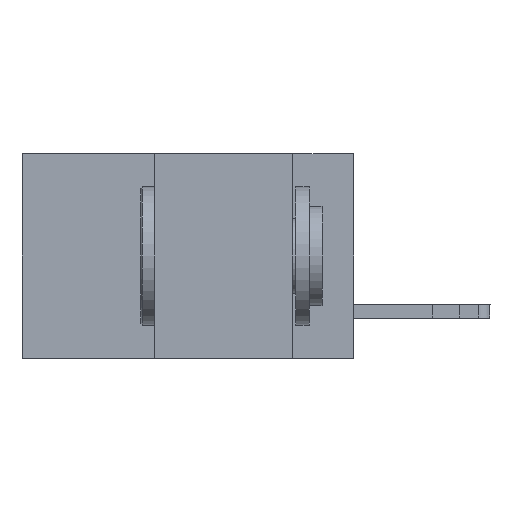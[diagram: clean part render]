
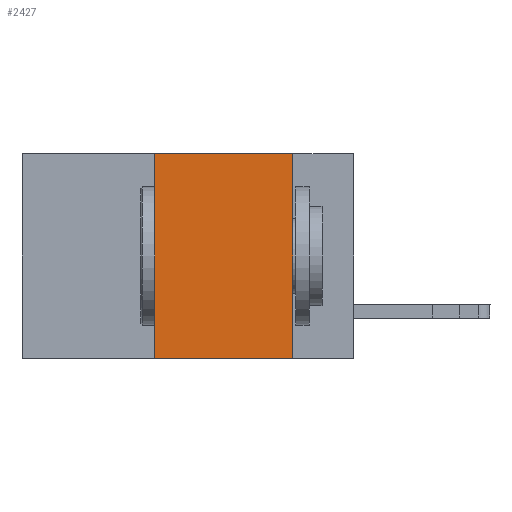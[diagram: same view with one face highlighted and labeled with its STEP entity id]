
A CAD part, left-side view. The second image highlights one B-rep face of the part: STEP entity #2427.
In plain terms, the highlighted planar face has unit normal (-1, 0, 0).
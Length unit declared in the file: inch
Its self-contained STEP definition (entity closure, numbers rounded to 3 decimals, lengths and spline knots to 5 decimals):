
#285 = DIRECTION ( 'NONE',  ( 0., 0., -1. ) ) ;
#447 = CARTESIAN_POINT ( 'NONE',  ( 0., 0.6, 0. ) ) ;
#644 = DIRECTION ( 'NONE',  ( 0., -1., 0. ) ) ;
#1502 = CARTESIAN_POINT ( 'NONE',  ( 0., 0.36, 0. ) ) ;
#1856 = EDGE_CURVE ( 'NONE', #11914, #11080, #3003, .T. ) ;
#2427 = ADVANCED_FACE ( 'NONE', ( #10348 ), #2671, .F. ) ;
#2671 = PLANE ( 'NONE',  #8887 ) ;
#3003 = LINE ( 'NONE', #12328, #4125 ) ;
#3534 = EDGE_LOOP ( 'NONE', ( #3798, #7673, #7021, #14537 ) ) ;
#3798 = ORIENTED_EDGE ( 'NONE', *, *, #1856, .F. ) ;
#3983 = EDGE_CURVE ( 'NONE', #14549, #11914, #4988, .T. ) ;
#4125 = VECTOR ( 'NONE', #285, 39.37008 ) ;
#4927 = CARTESIAN_POINT ( 'NONE',  ( 0., 0.36, -0.37 ) ) ;
#4988 = LINE ( 'NONE', #14996, #9188 ) ;
#7021 = ORIENTED_EDGE ( 'NONE', *, *, #10661, .F. ) ;
#7146 = DIRECTION ( 'NONE',  ( 0., 0., -1. ) ) ;
#7444 = CARTESIAN_POINT ( 'NONE',  ( 0., 0.11, -0.37 ) ) ;
#7673 = ORIENTED_EDGE ( 'NONE', *, *, #3983, .F. ) ;
#7869 = DIRECTION ( 'NONE',  ( 1., 0., 0. ) ) ;
#8065 = DIRECTION ( 'NONE',  ( 0., 0., 1. ) ) ;
#8155 = CARTESIAN_POINT ( 'NONE',  ( 0., 0.36, 0. ) ) ;
#8887 = AXIS2_PLACEMENT_3D ( 'NONE', #447, #7869, #7146 ) ;
#9188 = VECTOR ( 'NONE', #644, 39.37008 ) ;
#10348 = FACE_OUTER_BOUND ( 'NONE', #3534, .T. ) ;
#10661 = EDGE_CURVE ( 'NONE', #11404, #14549, #15087, .T. ) ;
#10823 = CARTESIAN_POINT ( 'NONE',  ( 0., 0.6, -0.37 ) ) ;
#11080 = VERTEX_POINT ( 'NONE', #7444 ) ;
#11404 = VERTEX_POINT ( 'NONE', #4927 ) ;
#11609 = VECTOR ( 'NONE', #14323, 39.37008 ) ;
#11681 = CARTESIAN_POINT ( 'NONE',  ( 0., 0.11, 0. ) ) ;
#11914 = VERTEX_POINT ( 'NONE', #11681 ) ;
#12328 = CARTESIAN_POINT ( 'NONE',  ( 0., 0.11, 0. ) ) ;
#12907 = EDGE_CURVE ( 'NONE', #11404, #11080, #15212, .T. ) ;
#14299 = VECTOR ( 'NONE', #8065, 39.37008 ) ;
#14323 = DIRECTION ( 'NONE',  ( 0., -1., 0. ) ) ;
#14537 = ORIENTED_EDGE ( 'NONE', *, *, #12907, .T. ) ;
#14549 = VERTEX_POINT ( 'NONE', #1502 ) ;
#14996 = CARTESIAN_POINT ( 'NONE',  ( 0., 0.6, 0. ) ) ;
#15087 = LINE ( 'NONE', #8155, #14299 ) ;
#15212 = LINE ( 'NONE', #10823, #11609 ) ;
